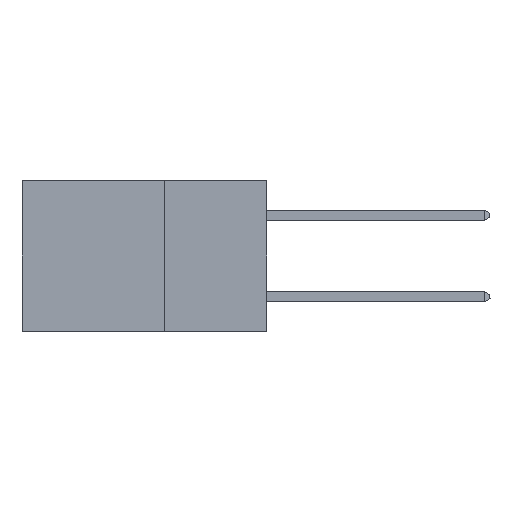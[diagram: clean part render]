
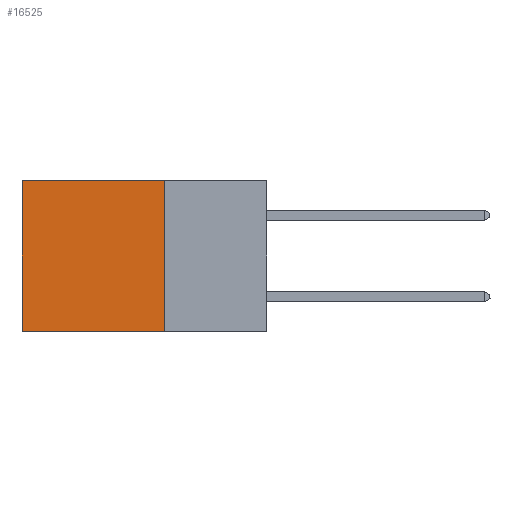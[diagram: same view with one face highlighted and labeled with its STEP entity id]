
A CAD part, left-side view. The second image highlights one B-rep face of the part: STEP entity #16525.
In plain terms, the highlighted planar face has unit normal (-1, 0, 0).
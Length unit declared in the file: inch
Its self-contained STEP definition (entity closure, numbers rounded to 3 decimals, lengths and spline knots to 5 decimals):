
#339 = CARTESIAN_POINT ( 'NONE',  ( 0.2875, 0.25, -0.37 ) ) ;
#936 = VECTOR ( 'NONE', #31618, 39.37008 ) ;
#4173 = LINE ( 'NONE', #24678, #6976 ) ;
#5443 = ORIENTED_EDGE ( 'NONE', *, *, #14703, .F. ) ;
#6029 = ORIENTED_EDGE ( 'NONE', *, *, #19849, .F. ) ;
#6976 = VECTOR ( 'NONE', #27113, 39.37008 ) ;
#8023 = VERTEX_POINT ( 'NONE', #23969 ) ;
#8511 = DIRECTION ( 'NONE',  ( 0., 0., -1. ) ) ;
#8853 = EDGE_LOOP ( 'NONE', ( #15066, #5443, #6029, #16608 ) ) ;
#14409 = DIRECTION ( 'NONE',  ( 1., 0., 0. ) ) ;
#14703 = EDGE_CURVE ( 'NONE', #19399, #32239, #28763, .T. ) ;
#15066 = ORIENTED_EDGE ( 'NONE', *, *, #18205, .T. ) ;
#16525 = ADVANCED_FACE ( 'NONE', ( #17407 ), #19827, .F. ) ;
#16608 = ORIENTED_EDGE ( 'NONE', *, *, #17733, .T. ) ;
#17407 = FACE_OUTER_BOUND ( 'NONE', #8853, .T. ) ;
#17733 = EDGE_CURVE ( 'NONE', #8023, #24951, #26471, .T. ) ;
#18205 = EDGE_CURVE ( 'NONE', #24951, #32239, #4173, .T. ) ;
#19076 = CARTESIAN_POINT ( 'NONE',  ( 0.2875, 0.6, -0.37 ) ) ;
#19225 = AXIS2_PLACEMENT_3D ( 'NONE', #24508, #14409, #22165 ) ;
#19399 = VERTEX_POINT ( 'NONE', #339 ) ;
#19827 = PLANE ( 'NONE',  #19225 ) ;
#19849 = EDGE_CURVE ( 'NONE', #8023, #19399, #32207, .T. ) ;
#20085 = VECTOR ( 'NONE', #25882, 39.37008 ) ;
#21929 = VECTOR ( 'NONE', #8511, 39.37008 ) ;
#22165 = DIRECTION ( 'NONE',  ( 0., 0., -1. ) ) ;
#23802 = CARTESIAN_POINT ( 'NONE',  ( 0.2875, 0.25, 0. ) ) ;
#23969 = CARTESIAN_POINT ( 'NONE',  ( 0.2875, 0.25, 0. ) ) ;
#24039 = CARTESIAN_POINT ( 'NONE',  ( 0.2875, 0.6, 0. ) ) ;
#24508 = CARTESIAN_POINT ( 'NONE',  ( 0.2875, 0.25, 0. ) ) ;
#24678 = CARTESIAN_POINT ( 'NONE',  ( 0.2875, 0.6, 0. ) ) ;
#24951 = VERTEX_POINT ( 'NONE', #24039 ) ;
#25882 = DIRECTION ( 'NONE',  ( 0., 1., 0. ) ) ;
#26471 = LINE ( 'NONE', #23802, #20085 ) ;
#27113 = DIRECTION ( 'NONE',  ( 0., 0., -1. ) ) ;
#28644 = CARTESIAN_POINT ( 'NONE',  ( 0.2875, 0.25, -0.37 ) ) ;
#28763 = LINE ( 'NONE', #28644, #936 ) ;
#31317 = CARTESIAN_POINT ( 'NONE',  ( 0.2875, 0.25, 0. ) ) ;
#31618 = DIRECTION ( 'NONE',  ( 0., 1., 0. ) ) ;
#32207 = LINE ( 'NONE', #31317, #21929 ) ;
#32239 = VERTEX_POINT ( 'NONE', #19076 ) ;
